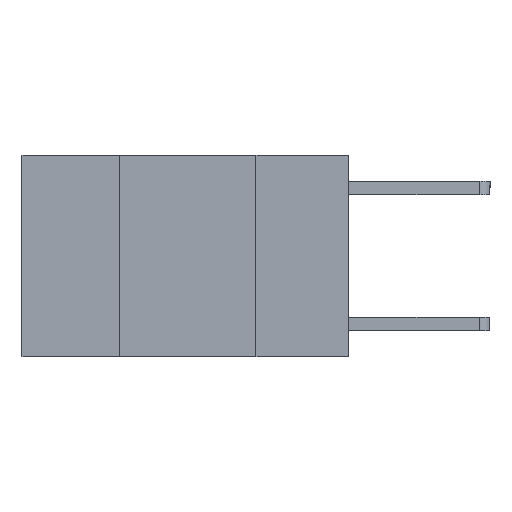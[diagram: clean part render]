
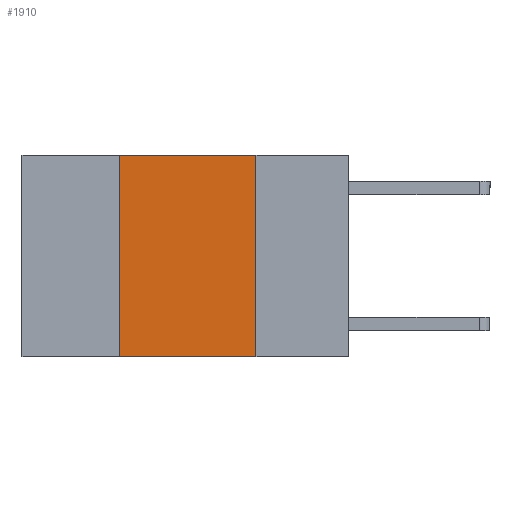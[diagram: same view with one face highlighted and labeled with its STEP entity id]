
A CAD part, left-side view. The second image highlights one B-rep face of the part: STEP entity #1910.
In plain terms, the highlighted planar face has unit normal (-1, 0, 0).
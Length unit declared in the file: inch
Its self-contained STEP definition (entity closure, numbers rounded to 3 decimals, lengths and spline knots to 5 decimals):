
#442 = DIRECTION ( 'NONE',  ( 0., 0., -1. ) ) ;
#542 = EDGE_CURVE ( 'NONE', #2783, #5330, #10829, .T. ) ;
#860 = AXIS2_PLACEMENT_3D ( 'NONE', #4921, #11144, #4808 ) ;
#1380 = CARTESIAN_POINT ( 'NONE',  ( 0., 0.17, 0. ) ) ;
#1728 = ORIENTED_EDGE ( 'NONE', *, *, #10557, .T. ) ;
#1910 = ADVANCED_FACE ( 'NONE', ( #2284 ), #9198, .F. ) ;
#2284 = FACE_OUTER_BOUND ( 'NONE', #11522, .T. ) ;
#2291 = DIRECTION ( 'NONE',  ( 0., -1., 0. ) ) ;
#2783 = VERTEX_POINT ( 'NONE', #9325 ) ;
#2872 = VECTOR ( 'NONE', #2291, 39.37008 ) ;
#2914 = CARTESIAN_POINT ( 'NONE',  ( 0., 0.6, 0. ) ) ;
#3024 = CARTESIAN_POINT ( 'NONE',  ( 0., 0.17, -0.37 ) ) ;
#3400 = CARTESIAN_POINT ( 'NONE',  ( 0., 0.42, -0.37 ) ) ;
#3496 = CARTESIAN_POINT ( 'NONE',  ( 0., 0.42, 0. ) ) ;
#4059 = LINE ( 'NONE', #4177, #4156 ) ;
#4156 = VECTOR ( 'NONE', #442, 39.37008 ) ;
#4177 = CARTESIAN_POINT ( 'NONE',  ( 0., 0.17, 0. ) ) ;
#4313 = DIRECTION ( 'NONE',  ( 0., 0., 1. ) ) ;
#4808 = DIRECTION ( 'NONE',  ( 0., 0., -1. ) ) ;
#4921 = CARTESIAN_POINT ( 'NONE',  ( 0., 0.6, 0. ) ) ;
#5330 = VERTEX_POINT ( 'NONE', #1380 ) ;
#5488 = EDGE_CURVE ( 'NONE', #8109, #2783, #8932, .T. ) ;
#5764 = LINE ( 'NONE', #9260, #2872 ) ;
#5823 = EDGE_CURVE ( 'NONE', #5330, #9517, #4059, .T. ) ;
#6320 = VECTOR ( 'NONE', #4313, 39.37008 ) ;
#7795 = ORIENTED_EDGE ( 'NONE', *, *, #5823, .F. ) ;
#8104 = ORIENTED_EDGE ( 'NONE', *, *, #5488, .F. ) ;
#8109 = VERTEX_POINT ( 'NONE', #3400 ) ;
#8932 = LINE ( 'NONE', #3496, #6320 ) ;
#9075 = ORIENTED_EDGE ( 'NONE', *, *, #542, .F. ) ;
#9198 = PLANE ( 'NONE',  #860 ) ;
#9260 = CARTESIAN_POINT ( 'NONE',  ( 0., 0.6, -0.37 ) ) ;
#9325 = CARTESIAN_POINT ( 'NONE',  ( 0., 0.42, 0. ) ) ;
#9517 = VERTEX_POINT ( 'NONE', #3024 ) ;
#10053 = DIRECTION ( 'NONE',  ( 0., -1., 0. ) ) ;
#10528 = VECTOR ( 'NONE', #10053, 39.37008 ) ;
#10557 = EDGE_CURVE ( 'NONE', #8109, #9517, #5764, .T. ) ;
#10829 = LINE ( 'NONE', #2914, #10528 ) ;
#11144 = DIRECTION ( 'NONE',  ( 1., 0., 0. ) ) ;
#11522 = EDGE_LOOP ( 'NONE', ( #7795, #9075, #8104, #1728 ) ) ;
